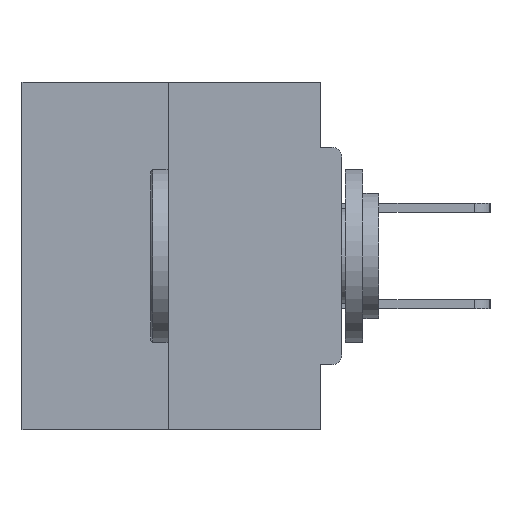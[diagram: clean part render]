
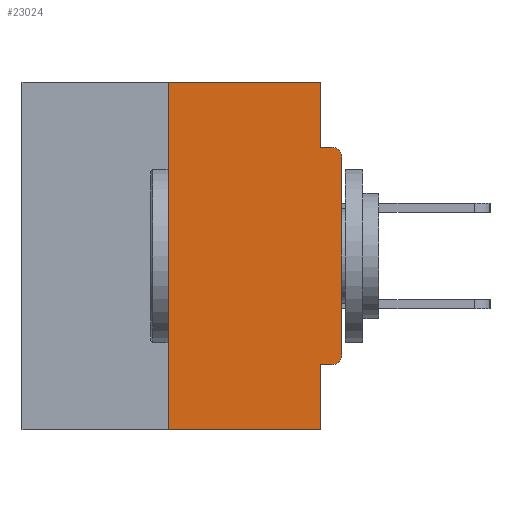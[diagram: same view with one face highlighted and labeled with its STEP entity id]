
A CAD part, left-side view. The second image highlights one B-rep face of the part: STEP entity #23024.
In plain terms, the highlighted planar face has unit normal (-1, 0, 0).
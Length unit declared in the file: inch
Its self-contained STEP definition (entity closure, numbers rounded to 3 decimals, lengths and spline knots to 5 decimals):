
#533 = CARTESIAN_POINT ( 'NONE',  ( 0., 0.031, 0. ) ) ;
#1308 = CARTESIAN_POINT ( 'NONE',  ( 0., 0., 0. ) ) ;
#2078 = LINE ( 'NONE', #33143, #15984 ) ;
#3050 = VERTEX_POINT ( 'NONE', #12512 ) ;
#3482 = CARTESIAN_POINT ( 'NONE',  ( 0., 0.25, 0. ) ) ;
#3791 = CARTESIAN_POINT ( 'NONE',  ( 0., 0.46, 0. ) ) ;
#3812 = VECTOR ( 'NONE', #7949, 39.37008 ) ;
#4713 = VECTOR ( 'NONE', #16289, 39.37008 ) ;
#4848 = ORIENTED_EDGE ( 'NONE', *, *, #30734, .F. ) ;
#5043 = ORIENTED_EDGE ( 'NONE', *, *, #25307, .T. ) ;
#5468 = VERTEX_POINT ( 'NONE', #3482 ) ;
#5980 = PLANE ( 'NONE',  #8545 ) ;
#6432 = LINE ( 'NONE', #1308, #27048 ) ;
#6645 = LINE ( 'NONE', #13104, #4713 ) ;
#7313 = ORIENTED_EDGE ( 'NONE', *, *, #20913, .T. ) ;
#7647 = CARTESIAN_POINT ( 'NONE',  ( 0., 0.031, -0.5 ) ) ;
#7691 = CARTESIAN_POINT ( 'NONE',  ( 0., 0.25, 0. ) ) ;
#7949 = DIRECTION ( 'NONE',  ( 0., 0., 1. ) ) ;
#8291 = DIRECTION ( 'NONE',  ( 0., -1., 0. ) ) ;
#8542 = CARTESIAN_POINT ( 'NONE',  ( 0., 0., -0.1085 ) ) ;
#8545 = AXIS2_PLACEMENT_3D ( 'NONE', #36928, #27709, #27443 ) ;
#8889 = DIRECTION ( 'NONE',  ( -1., 0., 0. ) ) ;
#9161 = ORIENTED_EDGE ( 'NONE', *, *, #9596, .F. ) ;
#9596 = EDGE_CURVE ( 'NONE', #15550, #5468, #23983, .T. ) ;
#9725 = VERTEX_POINT ( 'NONE', #17809 ) ;
#9872 = DIRECTION ( 'NONE',  ( 0., -1., 0. ) ) ;
#10077 = CARTESIAN_POINT ( 'NONE',  ( 0., 0.015, -0.0935 ) ) ;
#10433 = CARTESIAN_POINT ( 'NONE',  ( 0., 0.015, -0.4065 ) ) ;
#10608 = EDGE_LOOP ( 'NONE', ( #4848, #9161, #7313, #10744, #23127, #39601, #5043, #38373, #21763, #34782 ) ) ;
#10744 = ORIENTED_EDGE ( 'NONE', *, *, #30075, .F. ) ;
#12512 = CARTESIAN_POINT ( 'NONE',  ( 0., 0., -0.3915 ) ) ;
#12564 = DIRECTION ( 'NONE',  ( 0., 0., -1. ) ) ;
#13104 = CARTESIAN_POINT ( 'NONE',  ( 0., 0., -0.4065 ) ) ;
#14911 = CARTESIAN_POINT ( 'NONE',  ( 0., 0.015, -0.3915 ) ) ;
#15550 = VERTEX_POINT ( 'NONE', #32683 ) ;
#15755 = CIRCLE ( 'NONE', #16430, 0.015 ) ;
#15984 = VECTOR ( 'NONE', #8291, 39.37008 ) ;
#16256 = CARTESIAN_POINT ( 'NONE',  ( 0., 0.015, -0.1085 ) ) ;
#16289 = DIRECTION ( 'NONE',  ( 0., 1., 0. ) ) ;
#16430 = AXIS2_PLACEMENT_3D ( 'NONE', #14911, #8889, #24170 ) ;
#17809 = CARTESIAN_POINT ( 'NONE',  ( 0., 0.031, -0.5 ) ) ;
#18188 = VERTEX_POINT ( 'NONE', #10433 ) ;
#18514 = VECTOR ( 'NONE', #12564, 39.37008 ) ;
#19334 = DIRECTION ( 'NONE',  ( 0., 0., -1. ) ) ;
#19918 = LINE ( 'NONE', #34081, #18514 ) ;
#20913 = EDGE_CURVE ( 'NONE', #15550, #9725, #2078, .T. ) ;
#21763 = ORIENTED_EDGE ( 'NONE', *, *, #34365, .F. ) ;
#22569 = FACE_OUTER_BOUND ( 'NONE', #10608, .T. ) ;
#22766 = DIRECTION ( 'NONE',  ( 0., 0., 1. ) ) ;
#23024 = ADVANCED_FACE ( 'NONE', ( #22569 ), #5980, .F. ) ;
#23127 = ORIENTED_EDGE ( 'NONE', *, *, #29071, .F. ) ;
#23569 = LINE ( 'NONE', #35121, #31616 ) ;
#23983 = LINE ( 'NONE', #7691, #3812 ) ;
#23989 = EDGE_CURVE ( 'NONE', #18188, #3050, #15755, .T. ) ;
#24170 = DIRECTION ( 'NONE',  ( 0., 0., -1. ) ) ;
#25125 = DIRECTION ( 'NONE',  ( -1., 0., 0. ) ) ;
#25307 = EDGE_CURVE ( 'NONE', #3050, #36348, #6432, .T. ) ;
#25681 = VERTEX_POINT ( 'NONE', #10077 ) ;
#25953 = AXIS2_PLACEMENT_3D ( 'NONE', #16256, #25125, #19334 ) ;
#27048 = VECTOR ( 'NONE', #22766, 39.37008 ) ;
#27443 = DIRECTION ( 'NONE',  ( 0., 0., -1. ) ) ;
#27709 = DIRECTION ( 'NONE',  ( 1., 0., 0. ) ) ;
#29071 = EDGE_CURVE ( 'NONE', #18188, #33741, #6645, .T. ) ;
#29800 = CARTESIAN_POINT ( 'NONE',  ( 0., 0.031, -0.4065 ) ) ;
#30075 = EDGE_CURVE ( 'NONE', #33741, #9725, #33371, .T. ) ;
#30310 = EDGE_CURVE ( 'NONE', #32143, #35714, #19918, .T. ) ;
#30479 = VECTOR ( 'NONE', #35340, 39.37008 ) ;
#30734 = EDGE_CURVE ( 'NONE', #5468, #32143, #33758, .T. ) ;
#31616 = VECTOR ( 'NONE', #38350, 39.37008 ) ;
#32143 = VERTEX_POINT ( 'NONE', #533 ) ;
#32683 = CARTESIAN_POINT ( 'NONE',  ( 0., 0.25, -0.5 ) ) ;
#33143 = CARTESIAN_POINT ( 'NONE',  ( 0., 0.46, -0.5 ) ) ;
#33371 = LINE ( 'NONE', #7647, #30479 ) ;
#33741 = VERTEX_POINT ( 'NONE', #29800 ) ;
#33758 = LINE ( 'NONE', #3791, #35693 ) ;
#34081 = CARTESIAN_POINT ( 'NONE',  ( 0., 0.031, 0. ) ) ;
#34365 = EDGE_CURVE ( 'NONE', #35714, #25681, #23569, .T. ) ;
#34782 = ORIENTED_EDGE ( 'NONE', *, *, #30310, .F. ) ;
#35121 = CARTESIAN_POINT ( 'NONE',  ( 0., 0., -0.0935 ) ) ;
#35340 = DIRECTION ( 'NONE',  ( 0., 0., -1. ) ) ;
#35693 = VECTOR ( 'NONE', #9872, 39.37008 ) ;
#35714 = VERTEX_POINT ( 'NONE', #36122 ) ;
#36041 = EDGE_CURVE ( 'NONE', #36348, #25681, #36867, .T. ) ;
#36122 = CARTESIAN_POINT ( 'NONE',  ( 0., 0.031, -0.0935 ) ) ;
#36348 = VERTEX_POINT ( 'NONE', #8542 ) ;
#36867 = CIRCLE ( 'NONE', #25953, 0.015 ) ;
#36928 = CARTESIAN_POINT ( 'NONE',  ( 0., 0.46, 0. ) ) ;
#38350 = DIRECTION ( 'NONE',  ( 0., -1., 0. ) ) ;
#38373 = ORIENTED_EDGE ( 'NONE', *, *, #36041, .T. ) ;
#39601 = ORIENTED_EDGE ( 'NONE', *, *, #23989, .T. ) ;
